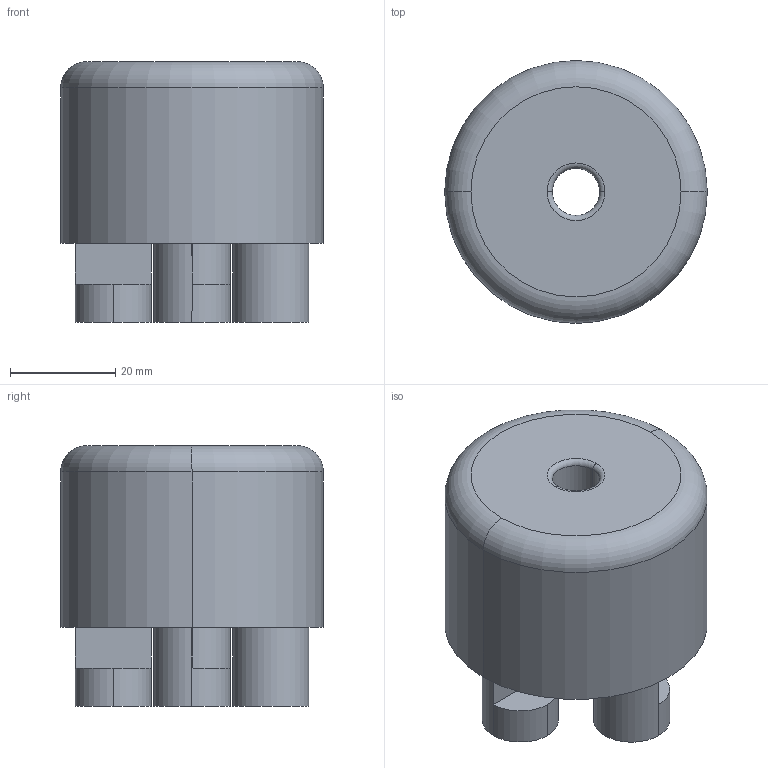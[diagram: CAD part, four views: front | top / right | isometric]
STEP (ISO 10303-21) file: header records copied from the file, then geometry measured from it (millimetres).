
FILE_DESCRIPTION (( 'STEP AP203' ), '1' );
FILE_NAME ('Barrel.STEP', '2013-08-28T12:52:42', ( '' ), ( '' ), 'SwSTEP 2.0', 'SolidWorks 2013', '' );
FILE_SCHEMA (( 'CONFIG_CONTROL_DESIGN' ));
Length unit declared in the file: millimetre
Products named in the file (1): Barrel
Bounding box: 50 x 50 x 49.6 mm (x, y, z)
Volume: 72146.7 mm3; surface area: 13015 mm2
Topology: 1 solids, 1 shells, 40 faces, 85 edges, 52 vertices
Faces by surface type: cylinder 19, plane 15, torus 6
Entity records: 1170 total; most frequent: DIRECTION 217, CARTESIAN_POINT 178, ORIENTED_EDGE 170, AXIS2_PLACEMENT_3D 91, EDGE_CURVE 85, VERTEX_POINT 52, CIRCLE 50, EDGE_LOOP 47
